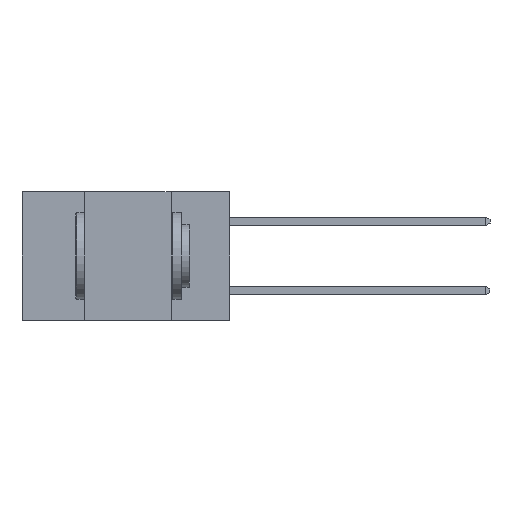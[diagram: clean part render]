
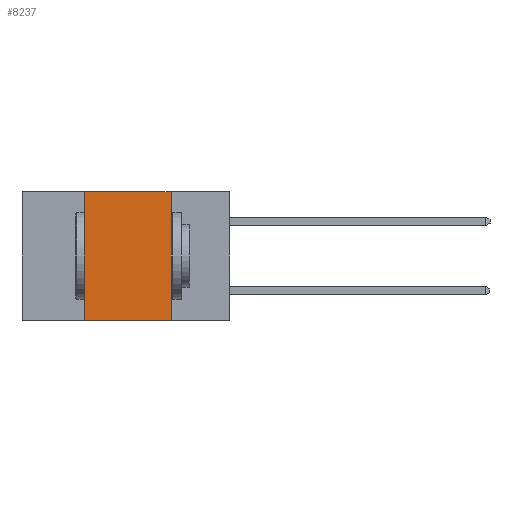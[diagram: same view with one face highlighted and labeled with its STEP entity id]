
A CAD part, left-side view. The second image highlights one B-rep face of the part: STEP entity #8237.
In plain terms, the highlighted planar face has unit normal (-1, 0, 0).
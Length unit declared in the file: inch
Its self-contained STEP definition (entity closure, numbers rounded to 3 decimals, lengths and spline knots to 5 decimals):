
#27 = EDGE_CURVE ( 'NONE', #12725, #8472, #7197, .T. ) ;
#824 = CARTESIAN_POINT ( 'NONE',  ( 0., 0.17, 0. ) ) ;
#910 = EDGE_CURVE ( 'NONE', #12725, #5370, #22812, .T. ) ;
#3275 = EDGE_CURVE ( 'NONE', #3432, #8472, #7038, .T. ) ;
#3432 = VERTEX_POINT ( 'NONE', #824 ) ;
#4014 = AXIS2_PLACEMENT_3D ( 'NONE', #11562, #18906, #7959 ) ;
#4259 = CARTESIAN_POINT ( 'NONE',  ( 0., 0.6, -0.37 ) ) ;
#4676 = ORIENTED_EDGE ( 'NONE', *, *, #27, .T. ) ;
#5370 = VERTEX_POINT ( 'NONE', #18133 ) ;
#5576 = LINE ( 'NONE', #14117, #14716 ) ;
#6690 = ORIENTED_EDGE ( 'NONE', *, *, #3275, .F. ) ;
#7038 = LINE ( 'NONE', #11543, #16205 ) ;
#7197 = LINE ( 'NONE', #4259, #16936 ) ;
#7825 = ORIENTED_EDGE ( 'NONE', *, *, #8469, .F. ) ;
#7959 = DIRECTION ( 'NONE',  ( 0., 0., -1. ) ) ;
#8237 = ADVANCED_FACE ( 'NONE', ( #10160 ), #9725, .F. ) ;
#8469 = EDGE_CURVE ( 'NONE', #5370, #3432, #5576, .T. ) ;
#8472 = VERTEX_POINT ( 'NONE', #12283 ) ;
#9725 = PLANE ( 'NONE',  #4014 ) ;
#10160 = FACE_OUTER_BOUND ( 'NONE', #17508, .T. ) ;
#10230 = DIRECTION ( 'NONE',  ( 0., 0., 1. ) ) ;
#11543 = CARTESIAN_POINT ( 'NONE',  ( 0., 0.17, 0. ) ) ;
#11562 = CARTESIAN_POINT ( 'NONE',  ( 0., 0.6, 0. ) ) ;
#12283 = CARTESIAN_POINT ( 'NONE',  ( 0., 0.17, -0.37 ) ) ;
#12725 = VERTEX_POINT ( 'NONE', #15430 ) ;
#13154 = VECTOR ( 'NONE', #10230, 39.37008 ) ;
#13254 = ORIENTED_EDGE ( 'NONE', *, *, #910, .F. ) ;
#14117 = CARTESIAN_POINT ( 'NONE',  ( 0., 0.6, 0. ) ) ;
#14716 = VECTOR ( 'NONE', #15962, 39.37008 ) ;
#15430 = CARTESIAN_POINT ( 'NONE',  ( 0., 0.42, -0.37 ) ) ;
#15962 = DIRECTION ( 'NONE',  ( 0., -1., 0. ) ) ;
#15995 = DIRECTION ( 'NONE',  ( 0., 0., -1. ) ) ;
#16205 = VECTOR ( 'NONE', #15995, 39.37008 ) ;
#16936 = VECTOR ( 'NONE', #21749, 39.37008 ) ;
#17508 = EDGE_LOOP ( 'NONE', ( #6690, #7825, #13254, #4676 ) ) ;
#18133 = CARTESIAN_POINT ( 'NONE',  ( 0., 0.42, 0. ) ) ;
#18906 = DIRECTION ( 'NONE',  ( 1., 0., 0. ) ) ;
#20229 = CARTESIAN_POINT ( 'NONE',  ( 0., 0.42, 0. ) ) ;
#21749 = DIRECTION ( 'NONE',  ( 0., -1., 0. ) ) ;
#22812 = LINE ( 'NONE', #20229, #13154 ) ;
